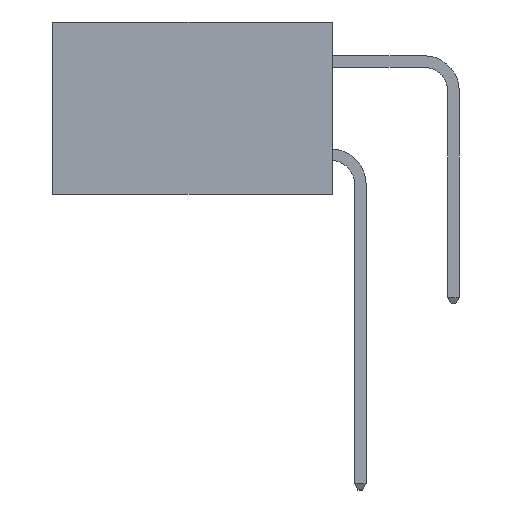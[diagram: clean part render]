
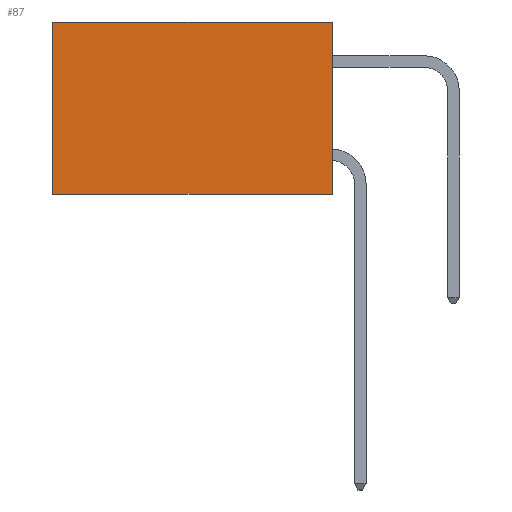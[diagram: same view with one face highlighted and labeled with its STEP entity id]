
A CAD part, left-side view. The second image highlights one B-rep face of the part: STEP entity #87.
In plain terms, the highlighted planar face has unit normal (-1, 0, 0).
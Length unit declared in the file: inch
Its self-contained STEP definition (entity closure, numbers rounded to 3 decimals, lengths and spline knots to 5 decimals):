
#56 = CARTESIAN_POINT ( 'NONE',  ( 0.2615, 0., -0.37 ) ) ;
#86 = DIRECTION ( 'NONE',  ( 1., 0., 0. ) ) ;
#87 = ADVANCED_FACE ( 'NONE', ( #2495 ), #6013, .F. ) ;
#243 = LINE ( 'NONE', #5483, #11336 ) ;
#1219 = VERTEX_POINT ( 'NONE', #9179 ) ;
#1899 = VECTOR ( 'NONE', #11881, 39.37008 ) ;
#1939 = VERTEX_POINT ( 'NONE', #12577 ) ;
#1998 = EDGE_LOOP ( 'NONE', ( #6389, #13038, #3239, #3961 ) ) ;
#2237 = LINE ( 'NONE', #11921, #1899 ) ;
#2495 = FACE_OUTER_BOUND ( 'NONE', #1998, .T. ) ;
#3166 = VECTOR ( 'NONE', #7323, 39.37008 ) ;
#3239 = ORIENTED_EDGE ( 'NONE', *, *, #10513, .F. ) ;
#3361 = DIRECTION ( 'NONE',  ( 0., 0., -1. ) ) ;
#3514 = LINE ( 'NONE', #9589, #3166 ) ;
#3841 = EDGE_CURVE ( 'NONE', #1939, #5757, #2237, .T. ) ;
#3961 = ORIENTED_EDGE ( 'NONE', *, *, #6017, .T. ) ;
#4334 = CARTESIAN_POINT ( 'NONE',  ( 0.2615, 0.6, 0. ) ) ;
#4451 = VECTOR ( 'NONE', #9187, 39.37008 ) ;
#5483 = CARTESIAN_POINT ( 'NONE',  ( 0.2615, 0., 0. ) ) ;
#5487 = DIRECTION ( 'NONE',  ( 0., 1., 0. ) ) ;
#5757 = VERTEX_POINT ( 'NONE', #8624 ) ;
#6013 = PLANE ( 'NONE',  #9714 ) ;
#6017 = EDGE_CURVE ( 'NONE', #1219, #7486, #243, .T. ) ;
#6389 = ORIENTED_EDGE ( 'NONE', *, *, #8500, .T. ) ;
#7323 = DIRECTION ( 'NONE',  ( 0., 0., -1. ) ) ;
#7486 = VERTEX_POINT ( 'NONE', #4334 ) ;
#8500 = EDGE_CURVE ( 'NONE', #7486, #5757, #3514, .T. ) ;
#8624 = CARTESIAN_POINT ( 'NONE',  ( 0.2615, 0.6, -0.37 ) ) ;
#9179 = CARTESIAN_POINT ( 'NONE',  ( 0.2615, 0., 0. ) ) ;
#9187 = DIRECTION ( 'NONE',  ( 0., 0., -1. ) ) ;
#9233 = CARTESIAN_POINT ( 'NONE',  ( 0.2615, 0., -0.37 ) ) ;
#9589 = CARTESIAN_POINT ( 'NONE',  ( 0.2615, 0.6, -0.37 ) ) ;
#9714 = AXIS2_PLACEMENT_3D ( 'NONE', #56, #86, #3361 ) ;
#10513 = EDGE_CURVE ( 'NONE', #1219, #1939, #12809, .T. ) ;
#11336 = VECTOR ( 'NONE', #5487, 39.37008 ) ;
#11881 = DIRECTION ( 'NONE',  ( 0., 1., 0. ) ) ;
#11921 = CARTESIAN_POINT ( 'NONE',  ( 0.2615, 0., -0.37 ) ) ;
#12577 = CARTESIAN_POINT ( 'NONE',  ( 0.2615, 0., -0.37 ) ) ;
#12809 = LINE ( 'NONE', #9233, #4451 ) ;
#13038 = ORIENTED_EDGE ( 'NONE', *, *, #3841, .F. ) ;
